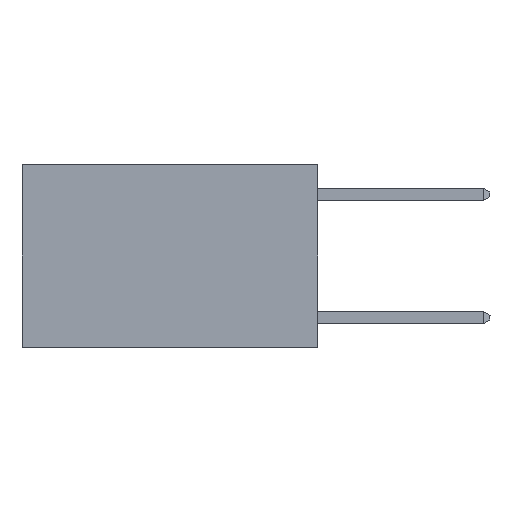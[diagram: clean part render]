
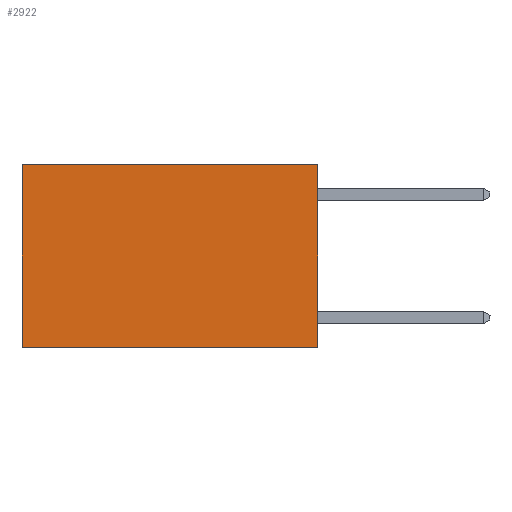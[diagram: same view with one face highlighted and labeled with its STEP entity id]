
A CAD part, left-side view. The second image highlights one B-rep face of the part: STEP entity #2922.
In plain terms, the highlighted planar face has unit normal (-1, 0, 0).
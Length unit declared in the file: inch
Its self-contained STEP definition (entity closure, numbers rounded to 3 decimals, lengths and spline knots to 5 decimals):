
#244 = LINE ( 'NONE', #10447, #10199 ) ;
#257 = VECTOR ( 'NONE', #4117, 39.37008 ) ;
#505 = DIRECTION ( 'NONE',  ( 0., 0., -1. ) ) ;
#947 = PLANE ( 'NONE',  #8413 ) ;
#1142 = FACE_OUTER_BOUND ( 'NONE', #5620, .T. ) ;
#2525 = VERTEX_POINT ( 'NONE', #10373 ) ;
#2922 = ADVANCED_FACE ( 'NONE', ( #1142 ), #947, .F. ) ;
#3037 = LINE ( 'NONE', #9657, #257 ) ;
#3353 = VERTEX_POINT ( 'NONE', #4450 ) ;
#3488 = DIRECTION ( 'NONE',  ( 0., 1., 0. ) ) ;
#3802 = LINE ( 'NONE', #8803, #9803 ) ;
#4117 = DIRECTION ( 'NONE',  ( 0., 1., 0. ) ) ;
#4281 = VERTEX_POINT ( 'NONE', #8763 ) ;
#4450 = CARTESIAN_POINT ( 'NONE',  ( 0.2625, 0., -0.37 ) ) ;
#4783 = ORIENTED_EDGE ( 'NONE', *, *, #7642, .T. ) ;
#5497 = DIRECTION ( 'NONE',  ( 0., 0., -1. ) ) ;
#5535 = VERTEX_POINT ( 'NONE', #7369 ) ;
#5620 = EDGE_LOOP ( 'NONE', ( #4783, #6002, #5829, #8126 ) ) ;
#5829 = ORIENTED_EDGE ( 'NONE', *, *, #10219, .F. ) ;
#6002 = ORIENTED_EDGE ( 'NONE', *, *, #8722, .F. ) ;
#6234 = CARTESIAN_POINT ( 'NONE',  ( 0.2625, 0.6, 0. ) ) ;
#6794 = DIRECTION ( 'NONE',  ( 0., 0., -1. ) ) ;
#7369 = CARTESIAN_POINT ( 'NONE',  ( 0.2625, 0.6, 0. ) ) ;
#7642 = EDGE_CURVE ( 'NONE', #5535, #4281, #10714, .T. ) ;
#8126 = ORIENTED_EDGE ( 'NONE', *, *, #11608, .T. ) ;
#8306 = DIRECTION ( 'NONE',  ( 1., 0., 0. ) ) ;
#8413 = AXIS2_PLACEMENT_3D ( 'NONE', #11148, #8306, #5497 ) ;
#8722 = EDGE_CURVE ( 'NONE', #3353, #4281, #3802, .T. ) ;
#8763 = CARTESIAN_POINT ( 'NONE',  ( 0.2625, 0.6, -0.37 ) ) ;
#8803 = CARTESIAN_POINT ( 'NONE',  ( 0.2625, 0., -0.37 ) ) ;
#9530 = VECTOR ( 'NONE', #505, 39.37008 ) ;
#9657 = CARTESIAN_POINT ( 'NONE',  ( 0.2625, 0., 0. ) ) ;
#9803 = VECTOR ( 'NONE', #3488, 39.37008 ) ;
#10199 = VECTOR ( 'NONE', #6794, 39.37008 ) ;
#10219 = EDGE_CURVE ( 'NONE', #2525, #3353, #244, .T. ) ;
#10373 = CARTESIAN_POINT ( 'NONE',  ( 0.2625, 0., 0. ) ) ;
#10447 = CARTESIAN_POINT ( 'NONE',  ( 0.2625, 0., 0. ) ) ;
#10714 = LINE ( 'NONE', #6234, #9530 ) ;
#11148 = CARTESIAN_POINT ( 'NONE',  ( 0.2625, 0., 0. ) ) ;
#11608 = EDGE_CURVE ( 'NONE', #2525, #5535, #3037, .T. ) ;
